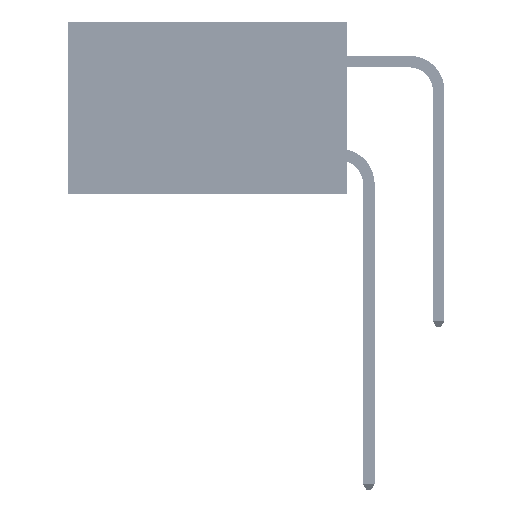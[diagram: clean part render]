
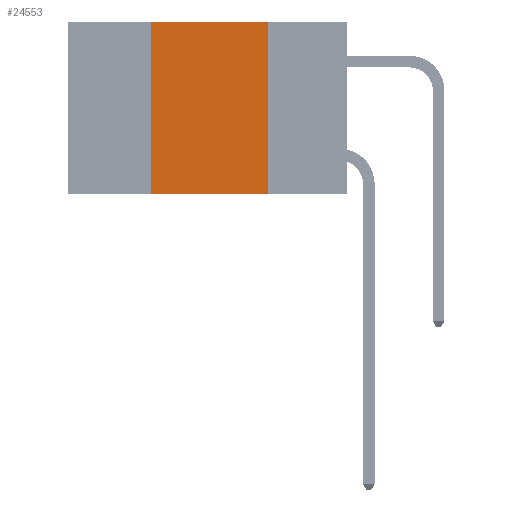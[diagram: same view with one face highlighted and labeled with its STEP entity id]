
A CAD part, left-side view. The second image highlights one B-rep face of the part: STEP entity #24553.
In plain terms, the highlighted planar face has unit normal (-1, 0, 0).
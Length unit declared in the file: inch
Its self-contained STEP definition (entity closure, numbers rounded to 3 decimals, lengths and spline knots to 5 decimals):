
#273 = DIRECTION ( 'NONE',  ( 0., 0., 1. ) ) ;
#2601 = DIRECTION ( 'NONE',  ( 0., 0., -1. ) ) ;
#3508 = VERTEX_POINT ( 'NONE', #18019 ) ;
#4696 = CARTESIAN_POINT ( 'NONE',  ( 0., 0.17, 0. ) ) ;
#5476 = EDGE_CURVE ( 'NONE', #3508, #12585, #47998, .T. ) ;
#6008 = EDGE_CURVE ( 'NONE', #12585, #27446, #24968, .T. ) ;
#6037 = FACE_OUTER_BOUND ( 'NONE', #8917, .T. ) ;
#7593 = VECTOR ( 'NONE', #48646, 39.37008 ) ;
#7763 = VECTOR ( 'NONE', #2601, 39.37008 ) ;
#8917 = EDGE_LOOP ( 'NONE', ( #46944, #11311, #23030, #51224 ) ) ;
#9130 = EDGE_CURVE ( 'NONE', #3508, #21935, #32536, .T. ) ;
#9393 = CARTESIAN_POINT ( 'NONE',  ( 0., 0.6, 0. ) ) ;
#9717 = CARTESIAN_POINT ( 'NONE',  ( 0., 0.6, 0. ) ) ;
#11311 = ORIENTED_EDGE ( 'NONE', *, *, #6008, .F. ) ;
#12585 = VERTEX_POINT ( 'NONE', #38483 ) ;
#13359 = DIRECTION ( 'NONE',  ( 0., -1., 0. ) ) ;
#18019 = CARTESIAN_POINT ( 'NONE',  ( 0., 0.42, -0.37 ) ) ;
#21164 = VECTOR ( 'NONE', #273, 39.37008 ) ;
#21854 = DIRECTION ( 'NONE',  ( 1., 0., 0. ) ) ;
#21935 = VERTEX_POINT ( 'NONE', #23321 ) ;
#23030 = ORIENTED_EDGE ( 'NONE', *, *, #5476, .F. ) ;
#23321 = CARTESIAN_POINT ( 'NONE',  ( 0., 0.17, -0.37 ) ) ;
#24553 = ADVANCED_FACE ( 'NONE', ( #6037 ), #30003, .F. ) ;
#24968 = LINE ( 'NONE', #9393, #44034 ) ;
#25038 = DIRECTION ( 'NONE',  ( 0., 0., -1. ) ) ;
#27446 = VERTEX_POINT ( 'NONE', #4696 ) ;
#28206 = CARTESIAN_POINT ( 'NONE',  ( 0., 0.42, 0. ) ) ;
#30003 = PLANE ( 'NONE',  #49331 ) ;
#32536 = LINE ( 'NONE', #37279, #7593 ) ;
#33727 = CARTESIAN_POINT ( 'NONE',  ( 0., 0.17, 0. ) ) ;
#34516 = LINE ( 'NONE', #33727, #7763 ) ;
#37279 = CARTESIAN_POINT ( 'NONE',  ( 0., 0.6, -0.37 ) ) ;
#38483 = CARTESIAN_POINT ( 'NONE',  ( 0., 0.42, 0. ) ) ;
#39829 = EDGE_CURVE ( 'NONE', #27446, #21935, #34516, .T. ) ;
#44034 = VECTOR ( 'NONE', #13359, 39.37008 ) ;
#46944 = ORIENTED_EDGE ( 'NONE', *, *, #39829, .F. ) ;
#47998 = LINE ( 'NONE', #28206, #21164 ) ;
#48646 = DIRECTION ( 'NONE',  ( 0., -1., 0. ) ) ;
#49331 = AXIS2_PLACEMENT_3D ( 'NONE', #9717, #21854, #25038 ) ;
#51224 = ORIENTED_EDGE ( 'NONE', *, *, #9130, .T. ) ;
